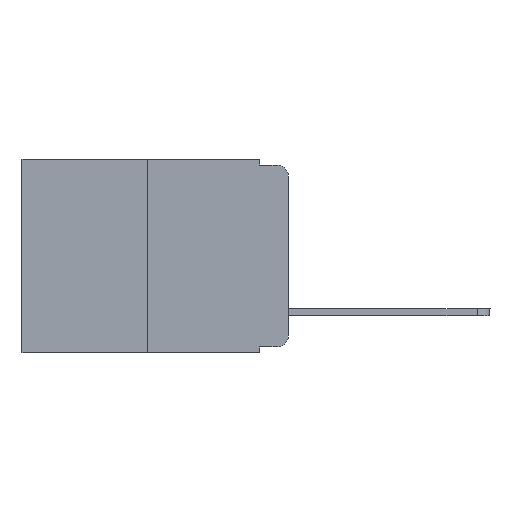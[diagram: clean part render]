
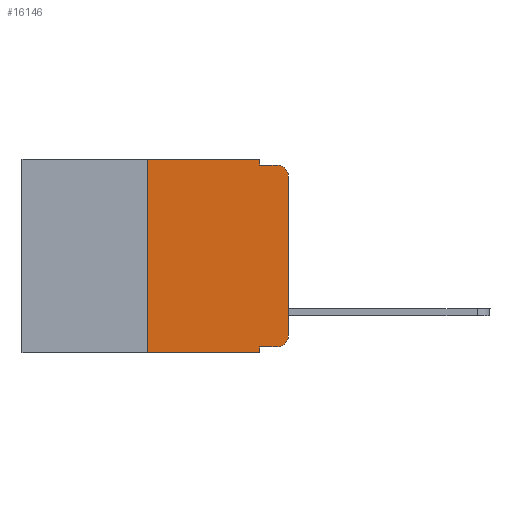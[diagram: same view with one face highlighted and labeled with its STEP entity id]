
A CAD part, left-side view. The second image highlights one B-rep face of the part: STEP entity #16146.
In plain terms, the highlighted planar face has unit normal (-1, 0, 0).
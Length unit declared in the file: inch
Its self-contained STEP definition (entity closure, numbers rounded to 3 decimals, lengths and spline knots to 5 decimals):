
#83 = LINE ( 'NONE', #3270, #12770 ) ;
#393 = CARTESIAN_POINT ( 'NONE',  ( 0., 0., -0.03 ) ) ;
#515 = CARTESIAN_POINT ( 'NONE',  ( 0., 0.051, -0.333 ) ) ;
#845 = DIRECTION ( 'NONE',  ( 0., 0., -1. ) ) ;
#1182 = DIRECTION ( 'NONE',  ( 0., -1., 0. ) ) ;
#1465 = CARTESIAN_POINT ( 'NONE',  ( 0., 0.25, 0. ) ) ;
#1588 = CARTESIAN_POINT ( 'NONE',  ( 0., 0.02, -0.313 ) ) ;
#1603 = EDGE_CURVE ( 'NONE', #7103, #17508, #9302, .T. ) ;
#1871 = FACE_OUTER_BOUND ( 'NONE', #6670, .T. ) ;
#1968 = ORIENTED_EDGE ( 'NONE', *, *, #17256, .F. ) ;
#2310 = CARTESIAN_POINT ( 'NONE',  ( 0., 0., -0.313 ) ) ;
#2451 = ORIENTED_EDGE ( 'NONE', *, *, #3296, .F. ) ;
#2465 = VERTEX_POINT ( 'NONE', #515 ) ;
#2837 = CARTESIAN_POINT ( 'NONE',  ( 0., 0.473, -0.343 ) ) ;
#3154 = DIRECTION ( 'NONE',  ( 0., 0., 1. ) ) ;
#3270 = CARTESIAN_POINT ( 'NONE',  ( 0., 0.051, -0.01 ) ) ;
#3296 = EDGE_CURVE ( 'NONE', #10809, #13310, #10716, .T. ) ;
#3542 = VECTOR ( 'NONE', #845, 39.37008 ) ;
#4456 = VECTOR ( 'NONE', #3154, 39.37008 ) ;
#4763 = EDGE_CURVE ( 'NONE', #13310, #18122, #8163, .T. ) ;
#4823 = VECTOR ( 'NONE', #7886, 39.37008 ) ;
#4838 = EDGE_CURVE ( 'NONE', #14442, #10809, #17741, .T. ) ;
#5132 = ORIENTED_EDGE ( 'NONE', *, *, #18954, .T. ) ;
#5643 = CARTESIAN_POINT ( 'NONE',  ( 0., 0.02, -0.333 ) ) ;
#5935 = ORIENTED_EDGE ( 'NONE', *, *, #18951, .T. ) ;
#6022 = LINE ( 'NONE', #2837, #12188 ) ;
#6256 = AXIS2_PLACEMENT_3D ( 'NONE', #17918, #16380, #6313 ) ;
#6313 = DIRECTION ( 'NONE',  ( 0., 0., -1. ) ) ;
#6524 = CARTESIAN_POINT ( 'NONE',  ( 0., 0.473, 0. ) ) ;
#6603 = ORIENTED_EDGE ( 'NONE', *, *, #10663, .T. ) ;
#6670 = EDGE_LOOP ( 'NONE', ( #5935, #7504, #1968, #6937, #2451, #12092, #5132, #8637, #6603, #7738 ) ) ;
#6937 = ORIENTED_EDGE ( 'NONE', *, *, #4763, .F. ) ;
#7083 = DIRECTION ( 'NONE',  ( -1., 0., 0. ) ) ;
#7099 = LINE ( 'NONE', #16013, #16089 ) ;
#7103 = VERTEX_POINT ( 'NONE', #393 ) ;
#7504 = ORIENTED_EDGE ( 'NONE', *, *, #1603, .T. ) ;
#7738 = ORIENTED_EDGE ( 'NONE', *, *, #12135, .T. ) ;
#7886 = DIRECTION ( 'NONE',  ( 0., -1., 0. ) ) ;
#8163 = LINE ( 'NONE', #14091, #3542 ) ;
#8537 = DIRECTION ( 'NONE',  ( -1., 0., 0. ) ) ;
#8557 = VECTOR ( 'NONE', #1182, 39.37008 ) ;
#8637 = ORIENTED_EDGE ( 'NONE', *, *, #14358, .F. ) ;
#8854 = DIRECTION ( 'NONE',  ( 0., 0., -1. ) ) ;
#8932 = CARTESIAN_POINT ( 'NONE',  ( 0., 0., 0. ) ) ;
#8977 = CARTESIAN_POINT ( 'NONE',  ( 0., 0.051, -0.01 ) ) ;
#9302 = CIRCLE ( 'NONE', #12670, 0.02 ) ;
#9341 = CIRCLE ( 'NONE', #9655, 0.02 ) ;
#9655 = AXIS2_PLACEMENT_3D ( 'NONE', #1588, #8537, #10176 ) ;
#9694 = VECTOR ( 'NONE', #11842, 39.37008 ) ;
#9768 = VERTEX_POINT ( 'NONE', #2310 ) ;
#9807 = DIRECTION ( 'NONE',  ( 0., 0., -1. ) ) ;
#10176 = DIRECTION ( 'NONE',  ( 0., 0., -1. ) ) ;
#10480 = PLANE ( 'NONE',  #6256 ) ;
#10663 = EDGE_CURVE ( 'NONE', #2465, #15978, #14423, .T. ) ;
#10716 = LINE ( 'NONE', #6524, #4823 ) ;
#10809 = VERTEX_POINT ( 'NONE', #1465 ) ;
#11653 = LINE ( 'NONE', #8932, #9694 ) ;
#11743 = CARTESIAN_POINT ( 'NONE',  ( 0., 0.051, 0. ) ) ;
#11842 = DIRECTION ( 'NONE',  ( 0., 0., 1. ) ) ;
#11940 = DIRECTION ( 'NONE',  ( 0., -1., 0. ) ) ;
#11965 = DIRECTION ( 'NONE',  ( 0., -1., 0. ) ) ;
#12092 = ORIENTED_EDGE ( 'NONE', *, *, #4838, .F. ) ;
#12135 = EDGE_CURVE ( 'NONE', #15978, #9768, #9341, .T. ) ;
#12183 = CARTESIAN_POINT ( 'NONE',  ( 0., 0.051, -0.343 ) ) ;
#12188 = VECTOR ( 'NONE', #11940, 39.37008 ) ;
#12446 = CARTESIAN_POINT ( 'NONE',  ( 0., 0.02, -0.01 ) ) ;
#12670 = AXIS2_PLACEMENT_3D ( 'NONE', #17451, #7083, #9807 ) ;
#12770 = VECTOR ( 'NONE', #11965, 39.37008 ) ;
#13310 = VERTEX_POINT ( 'NONE', #11743 ) ;
#14091 = CARTESIAN_POINT ( 'NONE',  ( 0., 0.051, 0. ) ) ;
#14358 = EDGE_CURVE ( 'NONE', #2465, #16935, #7099, .T. ) ;
#14423 = LINE ( 'NONE', #15964, #8557 ) ;
#14442 = VERTEX_POINT ( 'NONE', #16394 ) ;
#15964 = CARTESIAN_POINT ( 'NONE',  ( 0., 0.051, -0.333 ) ) ;
#15978 = VERTEX_POINT ( 'NONE', #5643 ) ;
#16013 = CARTESIAN_POINT ( 'NONE',  ( 0., 0.051, 0. ) ) ;
#16089 = VECTOR ( 'NONE', #8854, 39.37008 ) ;
#16146 = ADVANCED_FACE ( 'NONE', ( #1871 ), #10480, .F. ) ;
#16380 = DIRECTION ( 'NONE',  ( 1., 0., 0. ) ) ;
#16394 = CARTESIAN_POINT ( 'NONE',  ( 0., 0.25, -0.343 ) ) ;
#16935 = VERTEX_POINT ( 'NONE', #12183 ) ;
#17256 = EDGE_CURVE ( 'NONE', #18122, #17508, #83, .T. ) ;
#17451 = CARTESIAN_POINT ( 'NONE',  ( 0., 0.02, -0.03 ) ) ;
#17508 = VERTEX_POINT ( 'NONE', #12446 ) ;
#17741 = LINE ( 'NONE', #17843, #4456 ) ;
#17843 = CARTESIAN_POINT ( 'NONE',  ( 0., 0.25, 0. ) ) ;
#17918 = CARTESIAN_POINT ( 'NONE',  ( 0., 0.473, 0. ) ) ;
#18122 = VERTEX_POINT ( 'NONE', #8977 ) ;
#18951 = EDGE_CURVE ( 'NONE', #9768, #7103, #11653, .T. ) ;
#18954 = EDGE_CURVE ( 'NONE', #14442, #16935, #6022, .T. ) ;
